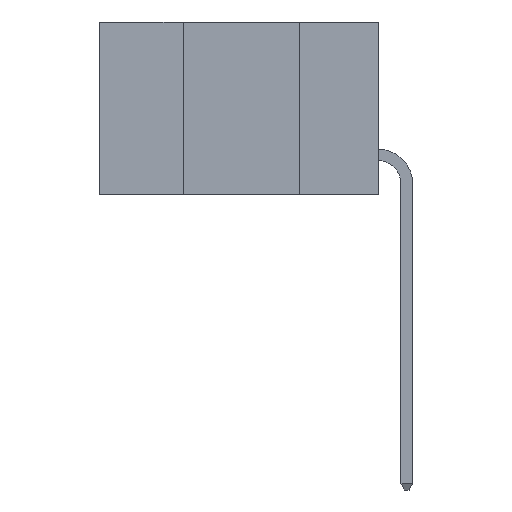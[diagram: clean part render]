
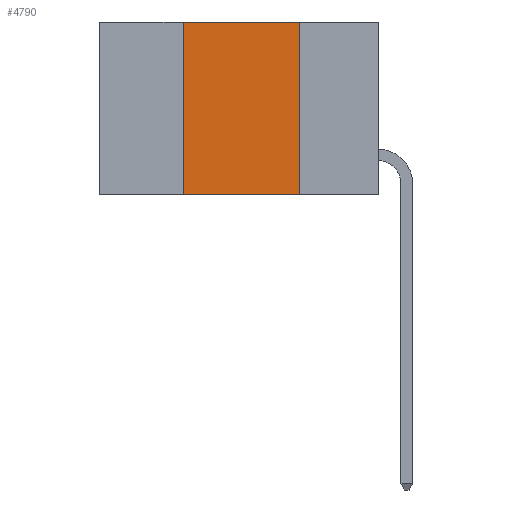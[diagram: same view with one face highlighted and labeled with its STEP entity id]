
A CAD part, left-side view. The second image highlights one B-rep face of the part: STEP entity #4790.
In plain terms, the highlighted planar face has unit normal (-1, 0, 0).
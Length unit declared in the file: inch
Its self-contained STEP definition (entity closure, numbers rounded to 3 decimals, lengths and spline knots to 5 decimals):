
#221 = VERTEX_POINT ( 'NONE', #9726 ) ;
#735 = ORIENTED_EDGE ( 'NONE', *, *, #4400, .F. ) ;
#809 = CARTESIAN_POINT ( 'NONE',  ( 0., 0.6, 0. ) ) ;
#1115 = VECTOR ( 'NONE', #4944, 39.37008 ) ;
#1437 = VERTEX_POINT ( 'NONE', #4259 ) ;
#1674 = CARTESIAN_POINT ( 'NONE',  ( 0., 0.17, 0. ) ) ;
#1762 = LINE ( 'NONE', #9032, #7347 ) ;
#1908 = EDGE_CURVE ( 'NONE', #1437, #9663, #5343, .T. ) ;
#2096 = EDGE_CURVE ( 'NONE', #4245, #221, #6102, .T. ) ;
#2582 = ORIENTED_EDGE ( 'NONE', *, *, #1908, .F. ) ;
#3736 = FACE_OUTER_BOUND ( 'NONE', #3844, .T. ) ;
#3844 = EDGE_LOOP ( 'NONE', ( #735, #2582, #4631, #6029 ) ) ;
#4027 = VECTOR ( 'NONE', #7317, 39.37008 ) ;
#4245 = VERTEX_POINT ( 'NONE', #8903 ) ;
#4259 = CARTESIAN_POINT ( 'NONE',  ( 0., 0.42, 0. ) ) ;
#4400 = EDGE_CURVE ( 'NONE', #9663, #221, #1762, .T. ) ;
#4631 = ORIENTED_EDGE ( 'NONE', *, *, #5129, .F. ) ;
#4790 = ADVANCED_FACE ( 'NONE', ( #3736 ), #6322, .F. ) ;
#4944 = DIRECTION ( 'NONE',  ( 0., 0., 1. ) ) ;
#4972 = DIRECTION ( 'NONE',  ( 0., -1., 0. ) ) ;
#4986 = CARTESIAN_POINT ( 'NONE',  ( 0., 0.42, -0.37 ) ) ;
#5112 = VECTOR ( 'NONE', #4972, 39.37008 ) ;
#5129 = EDGE_CURVE ( 'NONE', #4245, #1437, #7218, .T. ) ;
#5343 = LINE ( 'NONE', #809, #5112 ) ;
#6029 = ORIENTED_EDGE ( 'NONE', *, *, #2096, .T. ) ;
#6102 = LINE ( 'NONE', #7437, #4027 ) ;
#6322 = PLANE ( 'NONE',  #6475 ) ;
#6475 = AXIS2_PLACEMENT_3D ( 'NONE', #7397, #7393, #7385 ) ;
#7218 = LINE ( 'NONE', #4986, #1115 ) ;
#7317 = DIRECTION ( 'NONE',  ( 0., -1., 0. ) ) ;
#7347 = VECTOR ( 'NONE', #8930, 39.37008 ) ;
#7385 = DIRECTION ( 'NONE',  ( 0., 0., -1. ) ) ;
#7393 = DIRECTION ( 'NONE',  ( 1., 0., 0. ) ) ;
#7397 = CARTESIAN_POINT ( 'NONE',  ( 0., 0.6, 0. ) ) ;
#7437 = CARTESIAN_POINT ( 'NONE',  ( 0., 0.6, -0.37 ) ) ;
#8903 = CARTESIAN_POINT ( 'NONE',  ( 0., 0.42, -0.37 ) ) ;
#8930 = DIRECTION ( 'NONE',  ( 0., 0., -1. ) ) ;
#9032 = CARTESIAN_POINT ( 'NONE',  ( 0., 0.17, -0.37 ) ) ;
#9663 = VERTEX_POINT ( 'NONE', #1674 ) ;
#9726 = CARTESIAN_POINT ( 'NONE',  ( 0., 0.17, -0.37 ) ) ;
